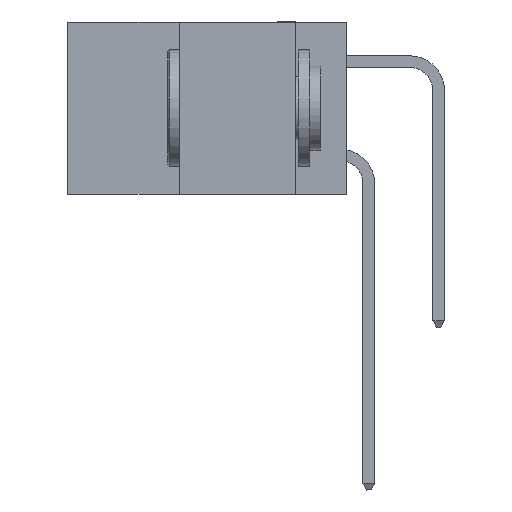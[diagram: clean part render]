
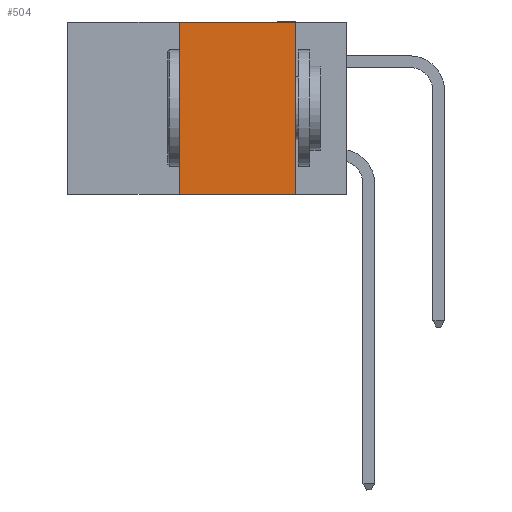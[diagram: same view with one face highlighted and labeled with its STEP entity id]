
A CAD part, left-side view. The second image highlights one B-rep face of the part: STEP entity #504.
In plain terms, the highlighted planar face has unit normal (-1, 0, 0).
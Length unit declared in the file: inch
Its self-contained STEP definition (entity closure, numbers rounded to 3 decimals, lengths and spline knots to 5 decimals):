
#66 = DIRECTION ( 'NONE',  ( 0., 0., -1. ) ) ;
#180 = VECTOR ( 'NONE', #8788, 39.37008 ) ;
#264 = CARTESIAN_POINT ( 'NONE',  ( 0., 0.36, 0. ) ) ;
#504 = ADVANCED_FACE ( 'NONE', ( #2924 ), #6812, .F. ) ;
#1381 = LINE ( 'NONE', #12665, #6297 ) ;
#2104 = LINE ( 'NONE', #6444, #10657 ) ;
#2276 = CARTESIAN_POINT ( 'NONE',  ( 0., 0.36, 0. ) ) ;
#2353 = ORIENTED_EDGE ( 'NONE', *, *, #11841, .F. ) ;
#2386 = DIRECTION ( 'NONE',  ( 0., -1., 0. ) ) ;
#2665 = EDGE_LOOP ( 'NONE', ( #10883, #2353, #10939, #3022 ) ) ;
#2924 = FACE_OUTER_BOUND ( 'NONE', #2665, .T. ) ;
#3022 = ORIENTED_EDGE ( 'NONE', *, *, #8345, .T. ) ;
#3140 = DIRECTION ( 'NONE',  ( 0., 0., 1. ) ) ;
#3258 = VERTEX_POINT ( 'NONE', #5585 ) ;
#3562 = LINE ( 'NONE', #11522, #180 ) ;
#5222 = LINE ( 'NONE', #264, #7955 ) ;
#5585 = CARTESIAN_POINT ( 'NONE',  ( 0., 0.36, -0.37 ) ) ;
#5950 = DIRECTION ( 'NONE',  ( 0., 0., -1. ) ) ;
#6056 = EDGE_CURVE ( 'NONE', #9170, #11833, #1381, .T. ) ;
#6297 = VECTOR ( 'NONE', #66, 39.37008 ) ;
#6305 = AXIS2_PLACEMENT_3D ( 'NONE', #8847, #11677, #5950 ) ;
#6444 = CARTESIAN_POINT ( 'NONE',  ( 0., 0.6, -0.37 ) ) ;
#6812 = PLANE ( 'NONE',  #6305 ) ;
#7062 = EDGE_CURVE ( 'NONE', #3258, #9746, #5222, .T. ) ;
#7353 = CARTESIAN_POINT ( 'NONE',  ( 0., 0.11, 0. ) ) ;
#7955 = VECTOR ( 'NONE', #3140, 39.37008 ) ;
#8345 = EDGE_CURVE ( 'NONE', #3258, #11833, #2104, .T. ) ;
#8788 = DIRECTION ( 'NONE',  ( 0., -1., 0. ) ) ;
#8847 = CARTESIAN_POINT ( 'NONE',  ( 0., 0.6, 0. ) ) ;
#9170 = VERTEX_POINT ( 'NONE', #7353 ) ;
#9209 = CARTESIAN_POINT ( 'NONE',  ( 0., 0.11, -0.37 ) ) ;
#9746 = VERTEX_POINT ( 'NONE', #2276 ) ;
#10657 = VECTOR ( 'NONE', #2386, 39.37008 ) ;
#10883 = ORIENTED_EDGE ( 'NONE', *, *, #6056, .F. ) ;
#10939 = ORIENTED_EDGE ( 'NONE', *, *, #7062, .F. ) ;
#11522 = CARTESIAN_POINT ( 'NONE',  ( 0., 0.6, 0. ) ) ;
#11677 = DIRECTION ( 'NONE',  ( 1., 0., 0. ) ) ;
#11833 = VERTEX_POINT ( 'NONE', #9209 ) ;
#11841 = EDGE_CURVE ( 'NONE', #9746, #9170, #3562, .T. ) ;
#12665 = CARTESIAN_POINT ( 'NONE',  ( 0., 0.11, 0. ) ) ;
